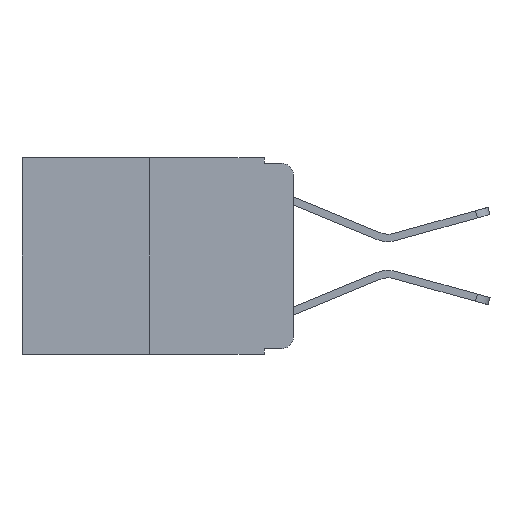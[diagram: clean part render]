
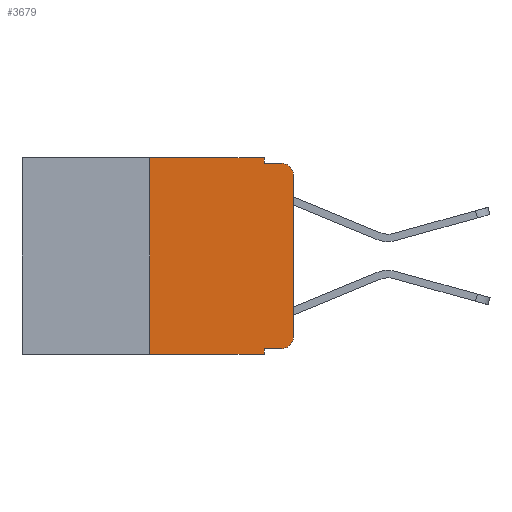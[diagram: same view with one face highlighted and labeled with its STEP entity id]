
A CAD part, left-side view. The second image highlights one B-rep face of the part: STEP entity #3679.
In plain terms, the highlighted planar face has unit normal (-1, 0, 0).
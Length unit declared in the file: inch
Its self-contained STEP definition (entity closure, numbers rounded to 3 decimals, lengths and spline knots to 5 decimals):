
#243 = EDGE_CURVE ( 'NONE', #20676, #17786, #22786, .T. ) ;
#283 = ORIENTED_EDGE ( 'NONE', *, *, #20841, .T. ) ;
#352 = ORIENTED_EDGE ( 'NONE', *, *, #17681, .T. ) ;
#396 = EDGE_LOOP ( 'NONE', ( #283, #352, #9912, #25019, #18519, #3392, #4973, #5718, #3659, #21955 ) ) ;
#600 = VECTOR ( 'NONE', #13604, 39.37008 ) ;
#1144 = DIRECTION ( 'NONE',  ( 0., 0., -1. ) ) ;
#1882 = VECTOR ( 'NONE', #22484, 39.37008 ) ;
#2069 = EDGE_CURVE ( 'NONE', #16472, #23881, #12956, .T. ) ;
#2103 = CARTESIAN_POINT ( 'NONE',  ( 0., 0., -0.313 ) ) ;
#2474 = CARTESIAN_POINT ( 'NONE',  ( 0., 0.051, -0.01 ) ) ;
#2571 = VECTOR ( 'NONE', #9089, 39.37008 ) ;
#2920 = DIRECTION ( 'NONE',  ( 0., 0., -1. ) ) ;
#3196 = CARTESIAN_POINT ( 'NONE',  ( 0., 0., 0. ) ) ;
#3392 = ORIENTED_EDGE ( 'NONE', *, *, #2069, .F. ) ;
#3500 = EDGE_CURVE ( 'NONE', #23881, #16536, #10753, .T. ) ;
#3633 = EDGE_CURVE ( 'NONE', #17662, #23629, #18061, .T. ) ;
#3659 = ORIENTED_EDGE ( 'NONE', *, *, #16152, .T. ) ;
#3679 = ADVANCED_FACE ( 'NONE', ( #7100 ), #16685, .F. ) ;
#4515 = AXIS2_PLACEMENT_3D ( 'NONE', #12871, #22872, #9630 ) ;
#4516 = VERTEX_POINT ( 'NONE', #2474 ) ;
#4961 = CARTESIAN_POINT ( 'NONE',  ( 0., 0.02, -0.03 ) ) ;
#4973 = ORIENTED_EDGE ( 'NONE', *, *, #11783, .T. ) ;
#5147 = DIRECTION ( 'NONE',  ( 0., 0., 1. ) ) ;
#5485 = CIRCLE ( 'NONE', #18360, 0.02 ) ;
#5718 = ORIENTED_EDGE ( 'NONE', *, *, #243, .F. ) ;
#5763 = LINE ( 'NONE', #3196, #23688 ) ;
#6080 = DIRECTION ( 'NONE',  ( 0., -1., 0. ) ) ;
#6312 = DIRECTION ( 'NONE',  ( 0., 0., -1. ) ) ;
#6947 = CARTESIAN_POINT ( 'NONE',  ( 0., 0.473, 0. ) ) ;
#7043 = VERTEX_POINT ( 'NONE', #19015 ) ;
#7100 = FACE_OUTER_BOUND ( 'NONE', #396, .T. ) ;
#7217 = DIRECTION ( 'NONE',  ( -1., 0., 0. ) ) ;
#7755 = CARTESIAN_POINT ( 'NONE',  ( 0., 0.051, -0.01 ) ) ;
#8550 = EDGE_CURVE ( 'NONE', #16536, #4516, #8682, .T. ) ;
#8682 = LINE ( 'NONE', #10414, #8974 ) ;
#8914 = CARTESIAN_POINT ( 'NONE',  ( 0., 0.25, 0. ) ) ;
#8974 = VECTOR ( 'NONE', #12147, 39.37008 ) ;
#9089 = DIRECTION ( 'NONE',  ( 0., 0., 1. ) ) ;
#9154 = VERTEX_POINT ( 'NONE', #15129 ) ;
#9168 = LINE ( 'NONE', #7755, #600 ) ;
#9630 = DIRECTION ( 'NONE',  ( 0., 0., -1. ) ) ;
#9912 = ORIENTED_EDGE ( 'NONE', *, *, #10981, .F. ) ;
#10414 = CARTESIAN_POINT ( 'NONE',  ( 0., 0.051, 0. ) ) ;
#10659 = CARTESIAN_POINT ( 'NONE',  ( 0., 0.051, 0. ) ) ;
#10753 = LINE ( 'NONE', #6947, #1882 ) ;
#10981 = EDGE_CURVE ( 'NONE', #4516, #9154, #9168, .T. ) ;
#11783 = EDGE_CURVE ( 'NONE', #16472, #17786, #19261, .T. ) ;
#12147 = DIRECTION ( 'NONE',  ( 0., 0., -1. ) ) ;
#12577 = VECTOR ( 'NONE', #6080, 39.37008 ) ;
#12790 = CARTESIAN_POINT ( 'NONE',  ( 0., 0.02, -0.313 ) ) ;
#12871 = CARTESIAN_POINT ( 'NONE',  ( 0., 0.473, 0. ) ) ;
#12956 = LINE ( 'NONE', #8914, #2571 ) ;
#12993 = CARTESIAN_POINT ( 'NONE',  ( 0., 0.051, -0.343 ) ) ;
#13604 = DIRECTION ( 'NONE',  ( 0., -1., 0. ) ) ;
#13655 = CARTESIAN_POINT ( 'NONE',  ( 0., 0.051, -0.333 ) ) ;
#13674 = AXIS2_PLACEMENT_3D ( 'NONE', #12790, #20498, #1144 ) ;
#14115 = VECTOR ( 'NONE', #14135, 39.37008 ) ;
#14135 = DIRECTION ( 'NONE',  ( 0., -1., 0. ) ) ;
#15129 = CARTESIAN_POINT ( 'NONE',  ( 0., 0.02, -0.01 ) ) ;
#16152 = EDGE_CURVE ( 'NONE', #20676, #17662, #20459, .T. ) ;
#16472 = VERTEX_POINT ( 'NONE', #20415 ) ;
#16536 = VERTEX_POINT ( 'NONE', #10659 ) ;
#16685 = PLANE ( 'NONE',  #4515 ) ;
#16893 = CARTESIAN_POINT ( 'NONE',  ( 0., 0.02, -0.333 ) ) ;
#17662 = VERTEX_POINT ( 'NONE', #16893 ) ;
#17681 = EDGE_CURVE ( 'NONE', #7043, #9154, #5485, .T. ) ;
#17786 = VERTEX_POINT ( 'NONE', #12993 ) ;
#17967 = CARTESIAN_POINT ( 'NONE',  ( 0., 0.473, -0.343 ) ) ;
#18055 = CARTESIAN_POINT ( 'NONE',  ( 0., 0.051, 0. ) ) ;
#18061 = CIRCLE ( 'NONE', #13674, 0.02 ) ;
#18213 = CARTESIAN_POINT ( 'NONE',  ( 0., 0.051, -0.333 ) ) ;
#18360 = AXIS2_PLACEMENT_3D ( 'NONE', #4961, #7217, #2920 ) ;
#18519 = ORIENTED_EDGE ( 'NONE', *, *, #3500, .F. ) ;
#19015 = CARTESIAN_POINT ( 'NONE',  ( 0., 0., -0.03 ) ) ;
#19261 = LINE ( 'NONE', #17967, #14115 ) ;
#20415 = CARTESIAN_POINT ( 'NONE',  ( 0., 0.25, -0.343 ) ) ;
#20459 = LINE ( 'NONE', #13655, #12577 ) ;
#20498 = DIRECTION ( 'NONE',  ( -1., 0., 0. ) ) ;
#20676 = VERTEX_POINT ( 'NONE', #18213 ) ;
#20841 = EDGE_CURVE ( 'NONE', #23629, #7043, #5763, .T. ) ;
#21955 = ORIENTED_EDGE ( 'NONE', *, *, #3633, .T. ) ;
#22359 = CARTESIAN_POINT ( 'NONE',  ( 0., 0.25, 0. ) ) ;
#22484 = DIRECTION ( 'NONE',  ( 0., -1., 0. ) ) ;
#22786 = LINE ( 'NONE', #18055, #24898 ) ;
#22872 = DIRECTION ( 'NONE',  ( 1., 0., 0. ) ) ;
#23629 = VERTEX_POINT ( 'NONE', #2103 ) ;
#23688 = VECTOR ( 'NONE', #5147, 39.37008 ) ;
#23881 = VERTEX_POINT ( 'NONE', #22359 ) ;
#24898 = VECTOR ( 'NONE', #6312, 39.37008 ) ;
#25019 = ORIENTED_EDGE ( 'NONE', *, *, #8550, .F. ) ;
